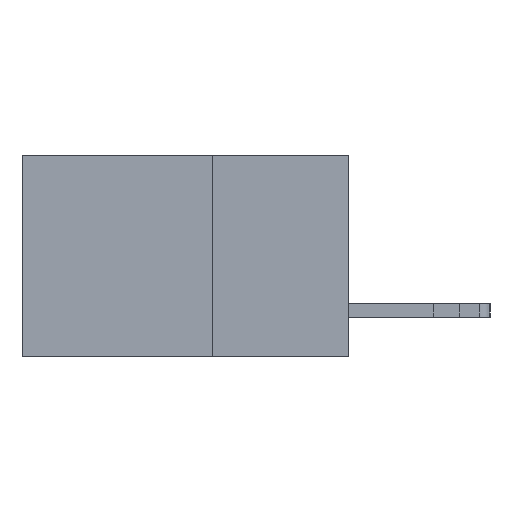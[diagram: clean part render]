
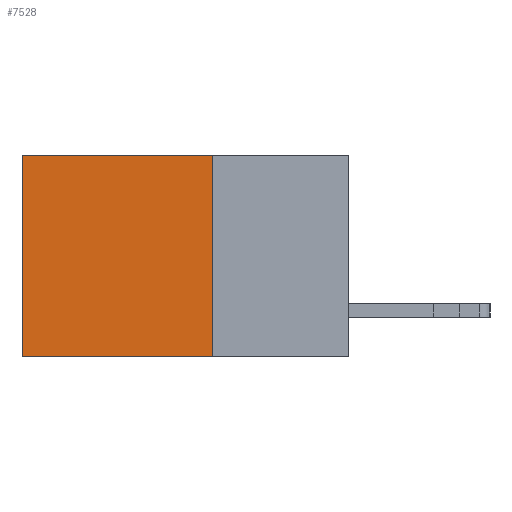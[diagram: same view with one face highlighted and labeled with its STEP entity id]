
A CAD part, left-side view. The second image highlights one B-rep face of the part: STEP entity #7528.
In plain terms, the highlighted planar face has unit normal (-1, 0, 0).
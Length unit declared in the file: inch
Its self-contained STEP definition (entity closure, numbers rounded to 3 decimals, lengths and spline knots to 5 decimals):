
#959 = CARTESIAN_POINT ( 'NONE',  ( 0.2615, 0.25, 0. ) ) ;
#2016 = DIRECTION ( 'NONE',  ( 0., 1., 0. ) ) ;
#2313 = CARTESIAN_POINT ( 'NONE',  ( 0.2615, 0.25, -0.37 ) ) ;
#2370 = CARTESIAN_POINT ( 'NONE',  ( 0.2615, 0.25, -0.37 ) ) ;
#5264 = ORIENTED_EDGE ( 'NONE', *, *, #6768, .T. ) ;
#5284 = VERTEX_POINT ( 'NONE', #15492 ) ;
#6368 = VECTOR ( 'NONE', #8601, 39.37008 ) ;
#6768 = EDGE_CURVE ( 'NONE', #10879, #5284, #16536, .T. ) ;
#7127 = VECTOR ( 'NONE', #2016, 39.37008 ) ;
#7528 = ADVANCED_FACE ( 'NONE', ( #7577 ), #9646, .F. ) ;
#7577 = FACE_OUTER_BOUND ( 'NONE', #15351, .T. ) ;
#8400 = EDGE_CURVE ( 'NONE', #11461, #5284, #10687, .T. ) ;
#8563 = VERTEX_POINT ( 'NONE', #11243 ) ;
#8601 = DIRECTION ( 'NONE',  ( 0., 0., -1. ) ) ;
#8793 = CARTESIAN_POINT ( 'NONE',  ( 0.2615, 0.6, -0.37 ) ) ;
#8926 = DIRECTION ( 'NONE',  ( 0., 0., -1. ) ) ;
#9083 = DIRECTION ( 'NONE',  ( 1., 0., 0. ) ) ;
#9163 = DIRECTION ( 'NONE',  ( 0., 0., -1. ) ) ;
#9167 = CARTESIAN_POINT ( 'NONE',  ( 0.2615, 0.25, -0.37 ) ) ;
#9309 = LINE ( 'NONE', #959, #12462 ) ;
#9317 = CARTESIAN_POINT ( 'NONE',  ( 0.2615, 0.25, -0.37 ) ) ;
#9445 = ORIENTED_EDGE ( 'NONE', *, *, #8400, .F. ) ;
#9646 = PLANE ( 'NONE',  #15933 ) ;
#9978 = VECTOR ( 'NONE', #9163, 39.37008 ) ;
#10687 = LINE ( 'NONE', #2313, #7127 ) ;
#10879 = VERTEX_POINT ( 'NONE', #14555 ) ;
#11243 = CARTESIAN_POINT ( 'NONE',  ( 0.2615, 0.25, 0. ) ) ;
#11461 = VERTEX_POINT ( 'NONE', #2370 ) ;
#12462 = VECTOR ( 'NONE', #14556, 39.37008 ) ;
#12650 = EDGE_CURVE ( 'NONE', #8563, #11461, #13169, .T. ) ;
#13169 = LINE ( 'NONE', #9167, #9978 ) ;
#13843 = ORIENTED_EDGE ( 'NONE', *, *, #14579, .T. ) ;
#14555 = CARTESIAN_POINT ( 'NONE',  ( 0.2615, 0.6, 0. ) ) ;
#14556 = DIRECTION ( 'NONE',  ( 0., 1., 0. ) ) ;
#14579 = EDGE_CURVE ( 'NONE', #8563, #10879, #9309, .T. ) ;
#15351 = EDGE_LOOP ( 'NONE', ( #5264, #9445, #15537, #13843 ) ) ;
#15492 = CARTESIAN_POINT ( 'NONE',  ( 0.2615, 0.6, -0.37 ) ) ;
#15537 = ORIENTED_EDGE ( 'NONE', *, *, #12650, .F. ) ;
#15933 = AXIS2_PLACEMENT_3D ( 'NONE', #9317, #9083, #8926 ) ;
#16536 = LINE ( 'NONE', #8793, #6368 ) ;
